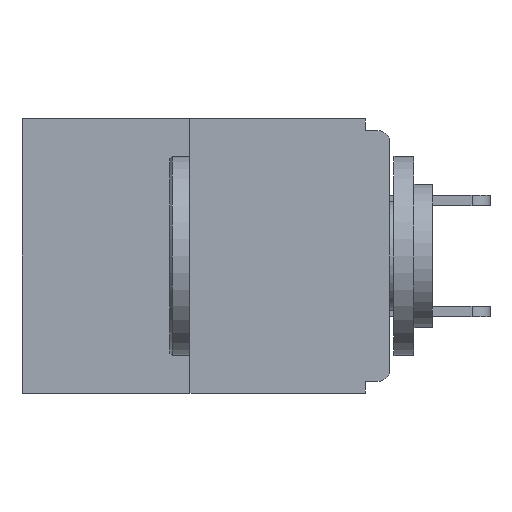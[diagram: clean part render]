
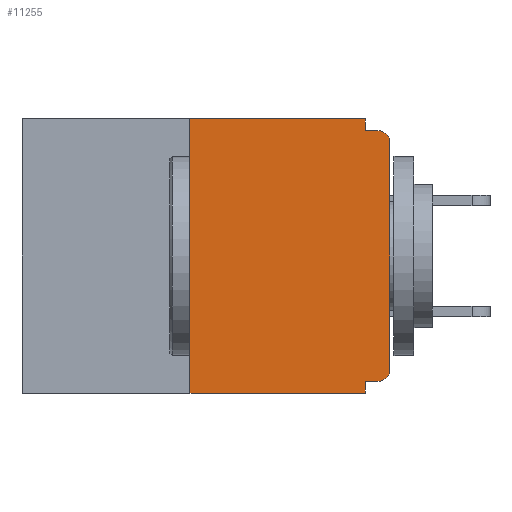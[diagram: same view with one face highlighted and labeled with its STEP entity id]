
A CAD part, left-side view. The second image highlights one B-rep face of the part: STEP entity #11255.
In plain terms, the highlighted planar face has unit normal (-1, 0, 0).
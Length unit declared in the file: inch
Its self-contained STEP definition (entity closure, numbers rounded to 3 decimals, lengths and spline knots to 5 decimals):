
#62 = CARTESIAN_POINT ( 'NONE',  ( 0., 0.031, -0.328 ) ) ;
#512 = VERTEX_POINT ( 'NONE', #15326 ) ;
#1132 = ORIENTED_EDGE ( 'NONE', *, *, #15892, .T. ) ;
#1638 = ORIENTED_EDGE ( 'NONE', *, *, #11941, .T. ) ;
#1750 = PLANE ( 'NONE',  #12375 ) ;
#1832 = CARTESIAN_POINT ( 'NONE',  ( 0., 0.031, 0. ) ) ;
#1906 = DIRECTION ( 'NONE',  ( 0., 0., -1. ) ) ;
#2579 = LINE ( 'NONE', #16635, #21780 ) ;
#3252 = VERTEX_POINT ( 'NONE', #23186 ) ;
#3523 = DIRECTION ( 'NONE',  ( 1., 0., 0. ) ) ;
#3537 = ORIENTED_EDGE ( 'NONE', *, *, #4164, .F. ) ;
#3646 = EDGE_LOOP ( 'NONE', ( #5786, #4859, #1132, #23185, #12603, #23233, #22867, #1638, #3537, #10395 ) ) ;
#3691 = CARTESIAN_POINT ( 'NONE',  ( 0., 0.015, -0.313 ) ) ;
#3999 = DIRECTION ( 'NONE',  ( 0., 0., -1. ) ) ;
#4164 = EDGE_CURVE ( 'NONE', #10367, #8956, #10154, .T. ) ;
#4189 = VECTOR ( 'NONE', #14231, 39.37008 ) ;
#4271 = DIRECTION ( 'NONE',  ( 0., -1., 0. ) ) ;
#4669 = VECTOR ( 'NONE', #4271, 39.37008 ) ;
#4859 = ORIENTED_EDGE ( 'NONE', *, *, #20259, .F. ) ;
#4899 = CARTESIAN_POINT ( 'NONE',  ( 0., 0.031, -0.343 ) ) ;
#5786 = ORIENTED_EDGE ( 'NONE', *, *, #15258, .F. ) ;
#5834 = DIRECTION ( 'NONE',  ( 0., 0., -1. ) ) ;
#6335 = LINE ( 'NONE', #1832, #22208 ) ;
#6353 = LINE ( 'NONE', #16999, #16816 ) ;
#6436 = CARTESIAN_POINT ( 'NONE',  ( 0., 0., -0.313 ) ) ;
#6926 = AXIS2_PLACEMENT_3D ( 'NONE', #14727, #14812, #3999 ) ;
#6992 = EDGE_CURVE ( 'NONE', #512, #10367, #6335, .T. ) ;
#7648 = VECTOR ( 'NONE', #22031, 39.37008 ) ;
#8956 = VERTEX_POINT ( 'NONE', #22581 ) ;
#8961 = LINE ( 'NONE', #20214, #15179 ) ;
#9194 = CARTESIAN_POINT ( 'NONE',  ( 0., 0.031, -0.015 ) ) ;
#9315 = EDGE_CURVE ( 'NONE', #21048, #18905, #2579, .T. ) ;
#9747 = DIRECTION ( 'NONE',  ( 0., 1., 0. ) ) ;
#9932 = CARTESIAN_POINT ( 'NONE',  ( 0., 0.25, 0. ) ) ;
#10154 = LINE ( 'NONE', #16631, #7648 ) ;
#10367 = VERTEX_POINT ( 'NONE', #9194 ) ;
#10395 = ORIENTED_EDGE ( 'NONE', *, *, #6992, .F. ) ;
#11255 = ADVANCED_FACE ( 'NONE', ( #21371 ), #1750, .F. ) ;
#11941 = EDGE_CURVE ( 'NONE', #21581, #8956, #19356, .T. ) ;
#12060 = CIRCLE ( 'NONE', #15752, 0.015 ) ;
#12375 = AXIS2_PLACEMENT_3D ( 'NONE', #19802, #3523, #18049 ) ;
#12603 = ORIENTED_EDGE ( 'NONE', *, *, #15133, .F. ) ;
#12671 = CARTESIAN_POINT ( 'NONE',  ( 0., 0.46, 0. ) ) ;
#12786 = VECTOR ( 'NONE', #13310, 39.37008 ) ;
#13310 = DIRECTION ( 'NONE',  ( 0., 0., 1. ) ) ;
#13576 = CARTESIAN_POINT ( 'NONE',  ( 0., 0.25, -0.343 ) ) ;
#14231 = DIRECTION ( 'NONE',  ( 0., -1., 0. ) ) ;
#14727 = CARTESIAN_POINT ( 'NONE',  ( 0., 0.015, -0.03 ) ) ;
#14812 = DIRECTION ( 'NONE',  ( -1., 0., 0. ) ) ;
#15099 = EDGE_CURVE ( 'NONE', #3252, #16898, #12060, .T. ) ;
#15133 = EDGE_CURVE ( 'NONE', #3252, #21048, #8961, .T. ) ;
#15179 = VECTOR ( 'NONE', #9747, 39.37008 ) ;
#15258 = EDGE_CURVE ( 'NONE', #22058, #512, #17690, .T. ) ;
#15326 = CARTESIAN_POINT ( 'NONE',  ( 0., 0.031, 0. ) ) ;
#15752 = AXIS2_PLACEMENT_3D ( 'NONE', #3691, #16311, #19978 ) ;
#15892 = EDGE_CURVE ( 'NONE', #17580, #18905, #18826, .T. ) ;
#16311 = DIRECTION ( 'NONE',  ( -1., 0., 0. ) ) ;
#16631 = CARTESIAN_POINT ( 'NONE',  ( 0., 0., -0.015 ) ) ;
#16635 = CARTESIAN_POINT ( 'NONE',  ( 0., 0.031, -0.343 ) ) ;
#16729 = LINE ( 'NONE', #22341, #12786 ) ;
#16816 = VECTOR ( 'NONE', #20662, 39.37008 ) ;
#16898 = VERTEX_POINT ( 'NONE', #6436 ) ;
#16999 = CARTESIAN_POINT ( 'NONE',  ( 0., 0.25, 0. ) ) ;
#17580 = VERTEX_POINT ( 'NONE', #13576 ) ;
#17690 = LINE ( 'NONE', #12671, #4189 ) ;
#17943 = CARTESIAN_POINT ( 'NONE',  ( 0., 0., -0.03 ) ) ;
#18049 = DIRECTION ( 'NONE',  ( 0., 0., -1. ) ) ;
#18663 = EDGE_CURVE ( 'NONE', #16898, #21581, #16729, .T. ) ;
#18826 = LINE ( 'NONE', #20406, #4669 ) ;
#18905 = VERTEX_POINT ( 'NONE', #4899 ) ;
#19356 = CIRCLE ( 'NONE', #6926, 0.015 ) ;
#19802 = CARTESIAN_POINT ( 'NONE',  ( 0., 0.46, 0. ) ) ;
#19978 = DIRECTION ( 'NONE',  ( 0., 0., -1. ) ) ;
#20214 = CARTESIAN_POINT ( 'NONE',  ( 0., 0., -0.328 ) ) ;
#20259 = EDGE_CURVE ( 'NONE', #17580, #22058, #6353, .T. ) ;
#20406 = CARTESIAN_POINT ( 'NONE',  ( 0., 0.46, -0.343 ) ) ;
#20662 = DIRECTION ( 'NONE',  ( 0., 0., 1. ) ) ;
#21048 = VERTEX_POINT ( 'NONE', #62 ) ;
#21371 = FACE_OUTER_BOUND ( 'NONE', #3646, .T. ) ;
#21581 = VERTEX_POINT ( 'NONE', #17943 ) ;
#21780 = VECTOR ( 'NONE', #5834, 39.37008 ) ;
#22031 = DIRECTION ( 'NONE',  ( 0., -1., 0. ) ) ;
#22058 = VERTEX_POINT ( 'NONE', #9932 ) ;
#22208 = VECTOR ( 'NONE', #1906, 39.37008 ) ;
#22341 = CARTESIAN_POINT ( 'NONE',  ( 0., 0., 0. ) ) ;
#22581 = CARTESIAN_POINT ( 'NONE',  ( 0., 0.015, -0.015 ) ) ;
#22867 = ORIENTED_EDGE ( 'NONE', *, *, #18663, .T. ) ;
#23185 = ORIENTED_EDGE ( 'NONE', *, *, #9315, .F. ) ;
#23186 = CARTESIAN_POINT ( 'NONE',  ( 0., 0.015, -0.328 ) ) ;
#23233 = ORIENTED_EDGE ( 'NONE', *, *, #15099, .T. ) ;
